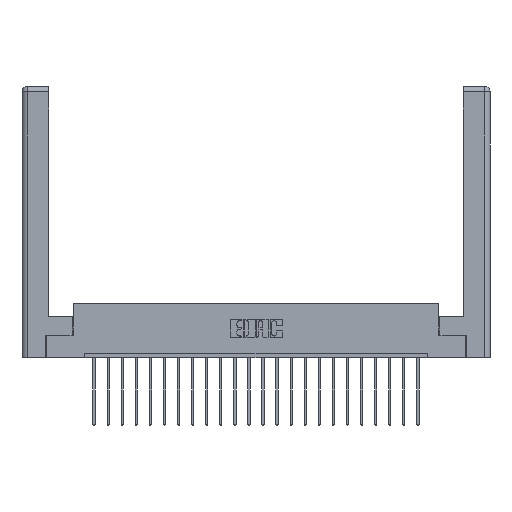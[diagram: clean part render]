
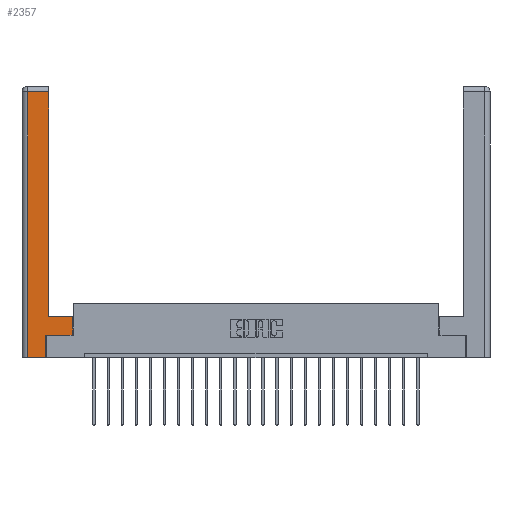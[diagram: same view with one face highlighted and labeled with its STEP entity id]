
A CAD part, top view. The second image highlights one B-rep face of the part: STEP entity #2357.
In plain terms, the highlighted planar face has unit normal (0, 0, 1).
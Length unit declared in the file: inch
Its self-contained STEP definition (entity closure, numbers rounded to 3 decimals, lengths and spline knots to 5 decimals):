
#906 = CARTESIAN_POINT ( 'NONE',  ( 0., 0., 0. ) ) ;
#2357 = ADVANCED_FACE ( 'NONE', ( #5183 ), #16624, .F. ) ;
#2771 = DIRECTION ( 'NONE',  ( 1., 0., 0. ) ) ;
#2805 = LINE ( 'NONE', #12190, #4722 ) ;
#2895 = CARTESIAN_POINT ( 'NONE',  ( 0.295, 3., 0. ) ) ;
#2980 = CARTESIAN_POINT ( 'NONE',  ( 0.265, 0., 0. ) ) ;
#2982 = EDGE_CURVE ( 'NONE', #10541, #18029, #20855, .T. ) ;
#3168 = LINE ( 'NONE', #5674, #3724 ) ;
#3394 = VECTOR ( 'NONE', #2771, 39.37008 ) ;
#3724 = VECTOR ( 'NONE', #18101, 39.37008 ) ;
#3929 = CARTESIAN_POINT ( 'NONE',  ( 0.295, 2.94, 0. ) ) ;
#4015 = EDGE_CURVE ( 'NONE', #6350, #10541, #3168, .T. ) ;
#4141 = DIRECTION ( 'NONE',  ( 1., 0., 0. ) ) ;
#4207 = LINE ( 'NONE', #21899, #3394 ) ;
#4264 = DIRECTION ( 'NONE',  ( -1., 0., 0. ) ) ;
#4630 = EDGE_CURVE ( 'NONE', #22133, #6350, #4207, .T. ) ;
#4722 = VECTOR ( 'NONE', #17208, 39.37008 ) ;
#5183 = FACE_OUTER_BOUND ( 'NONE', #21042, .T. ) ;
#5672 = ORIENTED_EDGE ( 'NONE', *, *, #20193, .T. ) ;
#5674 = CARTESIAN_POINT ( 'NONE',  ( 0.565, 0.45, 0. ) ) ;
#5877 = EDGE_CURVE ( 'NONE', #21766, #22133, #2805, .T. ) ;
#6154 = LINE ( 'NONE', #13011, #11659 ) ;
#6204 = DIRECTION ( 'NONE',  ( 0., -1., 0. ) ) ;
#6350 = VERTEX_POINT ( 'NONE', #8076 ) ;
#6904 = ORIENTED_EDGE ( 'NONE', *, *, #2982, .T. ) ;
#7093 = CARTESIAN_POINT ( 'NONE',  ( 0.0615, 2.94, 0. ) ) ;
#7217 = LINE ( 'NONE', #7696, #17145 ) ;
#7308 = DIRECTION ( 'NONE',  ( -1., 0., 0. ) ) ;
#7696 = CARTESIAN_POINT ( 'NONE',  ( 0.265, 0., 0. ) ) ;
#8047 = DIRECTION ( 'NONE',  ( 0., 0., -1. ) ) ;
#8076 = CARTESIAN_POINT ( 'NONE',  ( 0.565, 0.245, 0. ) ) ;
#9622 = CARTESIAN_POINT ( 'NONE',  ( 0.265, 0.245, 0. ) ) ;
#9720 = ORIENTED_EDGE ( 'NONE', *, *, #4015, .T. ) ;
#10541 = VERTEX_POINT ( 'NONE', #11387 ) ;
#11387 = CARTESIAN_POINT ( 'NONE',  ( 0.565, 0.45, 0. ) ) ;
#11659 = VECTOR ( 'NONE', #6204, 39.37008 ) ;
#11694 = DIRECTION ( 'NONE',  ( 0., 1., 0. ) ) ;
#12190 = CARTESIAN_POINT ( 'NONE',  ( 0.265, 0.245, 0. ) ) ;
#12672 = VERTEX_POINT ( 'NONE', #3929 ) ;
#12889 = LINE ( 'NONE', #2895, #14859 ) ;
#13011 = CARTESIAN_POINT ( 'NONE',  ( 0.0615, 0., 0. ) ) ;
#13130 = ORIENTED_EDGE ( 'NONE', *, *, #5877, .T. ) ;
#13140 = AXIS2_PLACEMENT_3D ( 'NONE', #906, #8047, #13216 ) ;
#13216 = DIRECTION ( 'NONE',  ( -1., 0., 0. ) ) ;
#13428 = VERTEX_POINT ( 'NONE', #21244 ) ;
#14197 = EDGE_CURVE ( 'NONE', #12672, #18051, #22804, .T. ) ;
#14211 = CARTESIAN_POINT ( 'NONE',  ( 0.0615, 2.94, 0. ) ) ;
#14480 = ORIENTED_EDGE ( 'NONE', *, *, #16956, .T. ) ;
#14775 = EDGE_CURVE ( 'NONE', #18029, #12672, #12889, .T. ) ;
#14837 = VECTOR ( 'NONE', #4264, 39.37008 ) ;
#14859 = VECTOR ( 'NONE', #11694, 39.37008 ) ;
#15923 = CARTESIAN_POINT ( 'NONE',  ( 0.295, 0.45, 0. ) ) ;
#15942 = ORIENTED_EDGE ( 'NONE', *, *, #4630, .T. ) ;
#16236 = VECTOR ( 'NONE', #7308, 39.37008 ) ;
#16406 = CARTESIAN_POINT ( 'NONE',  ( 0.295, 0.45, 0. ) ) ;
#16624 = PLANE ( 'NONE',  #13140 ) ;
#16825 = ORIENTED_EDGE ( 'NONE', *, *, #14775, .T. ) ;
#16956 = EDGE_CURVE ( 'NONE', #18051, #13428, #6154, .T. ) ;
#17145 = VECTOR ( 'NONE', #4141, 39.37008 ) ;
#17208 = DIRECTION ( 'NONE',  ( 0., 1., 0. ) ) ;
#18029 = VERTEX_POINT ( 'NONE', #15923 ) ;
#18051 = VERTEX_POINT ( 'NONE', #7093 ) ;
#18101 = DIRECTION ( 'NONE',  ( 0., 1., 0. ) ) ;
#20193 = EDGE_CURVE ( 'NONE', #13428, #21766, #7217, .T. ) ;
#20855 = LINE ( 'NONE', #16406, #14837 ) ;
#21042 = EDGE_LOOP ( 'NONE', ( #16825, #22633, #14480, #5672, #13130, #15942, #9720, #6904 ) ) ;
#21244 = CARTESIAN_POINT ( 'NONE',  ( 0.0615, 0., 0. ) ) ;
#21766 = VERTEX_POINT ( 'NONE', #2980 ) ;
#21899 = CARTESIAN_POINT ( 'NONE',  ( 0.565, 0.245, 0. ) ) ;
#22133 = VERTEX_POINT ( 'NONE', #9622 ) ;
#22633 = ORIENTED_EDGE ( 'NONE', *, *, #14197, .T. ) ;
#22804 = LINE ( 'NONE', #14211, #16236 ) ;
